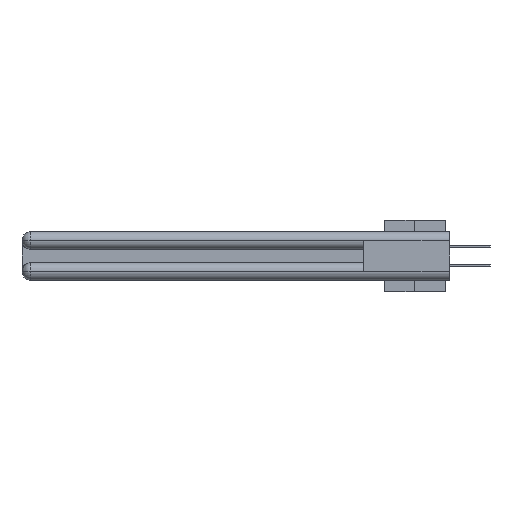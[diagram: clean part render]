
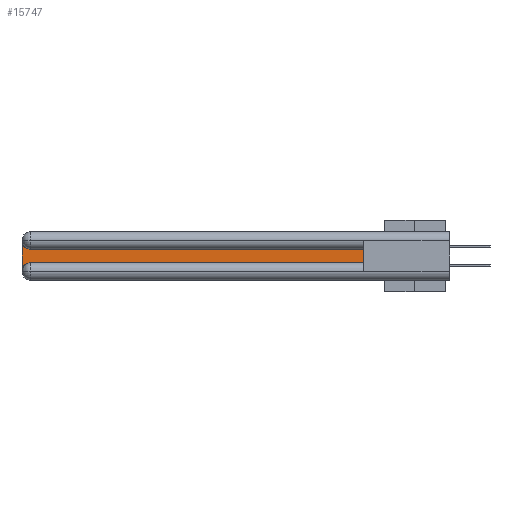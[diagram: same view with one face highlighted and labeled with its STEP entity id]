
A CAD part, left-side view. The second image highlights one B-rep face of the part: STEP entity #15747.
In plain terms, the highlighted planar face has unit normal (-1, 0, 0).
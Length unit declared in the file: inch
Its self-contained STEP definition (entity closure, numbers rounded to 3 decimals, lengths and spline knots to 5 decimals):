
#1293 = CARTESIAN_POINT ( 'NONE',  ( 0.075, 2.94, -0.1225 ) ) ;
#1344 = PLANE ( 'NONE',  #15946 ) ;
#1527 = CARTESIAN_POINT ( 'NONE',  ( 0.075, 0.6, -0.2175 ) ) ;
#1609 = ORIENTED_EDGE ( 'NONE', *, *, #6060, .T. ) ;
#2589 = LINE ( 'NONE', #14986, #30218 ) ;
#3573 = ORIENTED_EDGE ( 'NONE', *, *, #39446, .T. ) ;
#6060 = EDGE_CURVE ( 'NONE', #18123, #24484, #8317, .T. ) ;
#6578 = CIRCLE ( 'NONE', #34708, 0.06 ) ;
#7416 = DIRECTION ( 'NONE',  ( 1., 0., 0. ) ) ;
#8317 = LINE ( 'NONE', #22861, #13499 ) ;
#9323 = ORIENTED_EDGE ( 'NONE', *, *, #21779, .T. ) ;
#10701 = DIRECTION ( 'NONE',  ( 0., 0., -1. ) ) ;
#11265 = DIRECTION ( 'NONE',  ( 0., 1., 0. ) ) ;
#12602 = CARTESIAN_POINT ( 'NONE',  ( 0.075, 0.6, -0.2175 ) ) ;
#12966 = EDGE_LOOP ( 'NONE', ( #27182, #24997, #1609, #9323, #34183, #3573 ) ) ;
#13499 = VECTOR ( 'NONE', #16398, 39.37008 ) ;
#13878 = EDGE_CURVE ( 'NONE', #40778, #18123, #17558, .T. ) ;
#14558 = CARTESIAN_POINT ( 'NONE',  ( 0.075, 3., -0.1225 ) ) ;
#14986 = CARTESIAN_POINT ( 'NONE',  ( 0.075, 0.6, -0.1225 ) ) ;
#15263 = EDGE_CURVE ( 'NONE', #21460, #15389, #27378, .T. ) ;
#15389 = VERTEX_POINT ( 'NONE', #12602 ) ;
#15747 = ADVANCED_FACE ( 'NONE', ( #32891 ), #1344, .F. ) ;
#15883 = AXIS2_PLACEMENT_3D ( 'NONE', #20137, #7416, #10701 ) ;
#15946 = AXIS2_PLACEMENT_3D ( 'NONE', #14558, #34238, #27131 ) ;
#16398 = DIRECTION ( 'NONE',  ( 0., 0., -1. ) ) ;
#17558 = CIRCLE ( 'NONE', #15883, 0.06 ) ;
#18123 = VERTEX_POINT ( 'NONE', #40770 ) ;
#20137 = CARTESIAN_POINT ( 'NONE',  ( 0.075, 2.94, -0.0625 ) ) ;
#20323 = DIRECTION ( 'NONE',  ( 0., 0., 1. ) ) ;
#21089 = CARTESIAN_POINT ( 'NONE',  ( 0.075, 2.94, -0.2775 ) ) ;
#21334 = DIRECTION ( 'NONE',  ( 0., -1., 0. ) ) ;
#21460 = VERTEX_POINT ( 'NONE', #34124 ) ;
#21779 = EDGE_CURVE ( 'NONE', #24484, #21460, #6578, .T. ) ;
#22023 = CARTESIAN_POINT ( 'NONE',  ( 0.075, 0.6, -0.1225 ) ) ;
#22861 = CARTESIAN_POINT ( 'NONE',  ( 0.075, 3., -0.2175 ) ) ;
#24484 = VERTEX_POINT ( 'NONE', #25646 ) ;
#24997 = ORIENTED_EDGE ( 'NONE', *, *, #13878, .T. ) ;
#25646 = CARTESIAN_POINT ( 'NONE',  ( 0.075, 3., -0.2775 ) ) ;
#27131 = DIRECTION ( 'NONE',  ( 0., 0., -1. ) ) ;
#27182 = ORIENTED_EDGE ( 'NONE', *, *, #34929, .T. ) ;
#27378 = LINE ( 'NONE', #1527, #27837 ) ;
#27837 = VECTOR ( 'NONE', #21334, 39.37008 ) ;
#29215 = LINE ( 'NONE', #36729, #38952 ) ;
#30218 = VECTOR ( 'NONE', #11265, 39.37008 ) ;
#30652 = DIRECTION ( 'NONE',  ( 0., 0., -1. ) ) ;
#32891 = FACE_OUTER_BOUND ( 'NONE', #12966, .T. ) ;
#34124 = CARTESIAN_POINT ( 'NONE',  ( 0.075, 2.94, -0.2175 ) ) ;
#34183 = ORIENTED_EDGE ( 'NONE', *, *, #15263, .T. ) ;
#34238 = DIRECTION ( 'NONE',  ( 1., 0., 0. ) ) ;
#34708 = AXIS2_PLACEMENT_3D ( 'NONE', #21089, #40085, #30652 ) ;
#34929 = EDGE_CURVE ( 'NONE', #41585, #40778, #2589, .T. ) ;
#36729 = CARTESIAN_POINT ( 'NONE',  ( 0.075, 0.6, -0.2175 ) ) ;
#38952 = VECTOR ( 'NONE', #20323, 39.37008 ) ;
#39446 = EDGE_CURVE ( 'NONE', #15389, #41585, #29215, .T. ) ;
#40085 = DIRECTION ( 'NONE',  ( 1., 0., 0. ) ) ;
#40770 = CARTESIAN_POINT ( 'NONE',  ( 0.075, 3., -0.0625 ) ) ;
#40778 = VERTEX_POINT ( 'NONE', #1293 ) ;
#41585 = VERTEX_POINT ( 'NONE', #22023 ) ;
